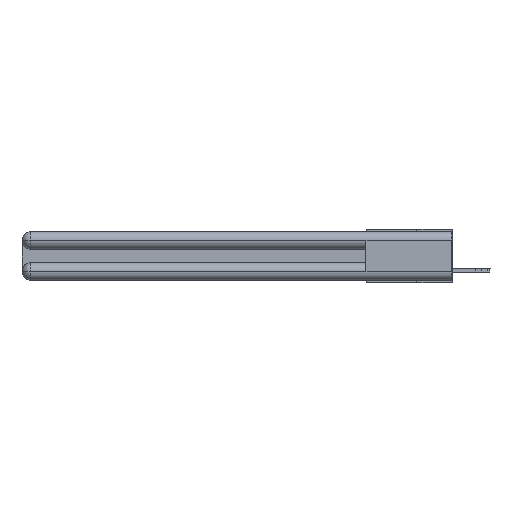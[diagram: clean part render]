
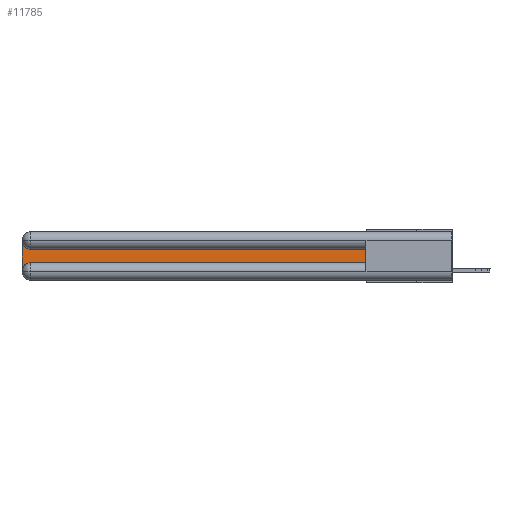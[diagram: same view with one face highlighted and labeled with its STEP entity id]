
A CAD part, left-side view. The second image highlights one B-rep face of the part: STEP entity #11785.
In plain terms, the highlighted planar face has unit normal (-1, 0, 0).
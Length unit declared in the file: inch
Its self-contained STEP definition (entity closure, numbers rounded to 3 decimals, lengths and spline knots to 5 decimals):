
#1414 = VERTEX_POINT ( 'NONE', #13036 ) ;
#1997 = LINE ( 'NONE', #21992, #21775 ) ;
#3199 = EDGE_CURVE ( 'NONE', #17450, #18612, #3644, .T. ) ;
#3342 = AXIS2_PLACEMENT_3D ( 'NONE', #25469, #17498, #21506 ) ;
#3433 = EDGE_LOOP ( 'NONE', ( #16272, #20812, #24108, #17010, #16637, #19248 ) ) ;
#3644 = LINE ( 'NONE', #16862, #15412 ) ;
#3791 = DIRECTION ( 'NONE',  ( 0., 0., -1. ) ) ;
#3910 = DIRECTION ( 'NONE',  ( 1., 0., 0. ) ) ;
#4842 = AXIS2_PLACEMENT_3D ( 'NONE', #20042, #3910, #5794 ) ;
#4911 = EDGE_CURVE ( 'NONE', #5305, #17450, #18140, .T. ) ;
#5305 = VERTEX_POINT ( 'NONE', #14785 ) ;
#5508 = CARTESIAN_POINT ( 'NONE',  ( 0.075, 2.94, -0.2775 ) ) ;
#5794 = DIRECTION ( 'NONE',  ( 0., 0., -1. ) ) ;
#6445 = CIRCLE ( 'NONE', #13655, 0.06 ) ;
#6840 = CARTESIAN_POINT ( 'NONE',  ( 0.075, 0.6, -0.2175 ) ) ;
#7050 = VERTEX_POINT ( 'NONE', #12999 ) ;
#8280 = VECTOR ( 'NONE', #10833, 39.37008 ) ;
#8893 = VECTOR ( 'NONE', #21657, 39.37008 ) ;
#9766 = PLANE ( 'NONE',  #4842 ) ;
#9778 = CARTESIAN_POINT ( 'NONE',  ( 0.075, 2.94, -0.2175 ) ) ;
#10819 = DIRECTION ( 'NONE',  ( 0., 1., 0. ) ) ;
#10833 = DIRECTION ( 'NONE',  ( 0., 0., 1. ) ) ;
#11087 = VERTEX_POINT ( 'NONE', #9778 ) ;
#11785 = ADVANCED_FACE ( 'NONE', ( #13609 ), #9766, .F. ) ;
#12999 = CARTESIAN_POINT ( 'NONE',  ( 0.075, 3., -0.0625 ) ) ;
#13036 = CARTESIAN_POINT ( 'NONE',  ( 0.075, 3., -0.2775 ) ) ;
#13304 = CARTESIAN_POINT ( 'NONE',  ( 0.075, 2.94, -0.1225 ) ) ;
#13609 = FACE_OUTER_BOUND ( 'NONE', #3433, .T. ) ;
#13655 = AXIS2_PLACEMENT_3D ( 'NONE', #5508, #25874, #15913 ) ;
#13924 = LINE ( 'NONE', #15565, #8893 ) ;
#14785 = CARTESIAN_POINT ( 'NONE',  ( 0.075, 0.6, -0.2175 ) ) ;
#15412 = VECTOR ( 'NONE', #10819, 39.37008 ) ;
#15565 = CARTESIAN_POINT ( 'NONE',  ( 0.075, 0.6, -0.2175 ) ) ;
#15913 = DIRECTION ( 'NONE',  ( 0., 0., -1. ) ) ;
#16272 = ORIENTED_EDGE ( 'NONE', *, *, #3199, .T. ) ;
#16637 = ORIENTED_EDGE ( 'NONE', *, *, #22277, .T. ) ;
#16862 = CARTESIAN_POINT ( 'NONE',  ( 0.075, 0.6, -0.1225 ) ) ;
#17010 = ORIENTED_EDGE ( 'NONE', *, *, #24891, .T. ) ;
#17450 = VERTEX_POINT ( 'NONE', #21426 ) ;
#17498 = DIRECTION ( 'NONE',  ( 1., 0., 0. ) ) ;
#18140 = LINE ( 'NONE', #6840, #8280 ) ;
#18612 = VERTEX_POINT ( 'NONE', #13304 ) ;
#19248 = ORIENTED_EDGE ( 'NONE', *, *, #4911, .T. ) ;
#19491 = EDGE_CURVE ( 'NONE', #7050, #1414, #1997, .T. ) ;
#20042 = CARTESIAN_POINT ( 'NONE',  ( 0.075, 3., -0.1225 ) ) ;
#20812 = ORIENTED_EDGE ( 'NONE', *, *, #21091, .T. ) ;
#21055 = CIRCLE ( 'NONE', #3342, 0.06 ) ;
#21091 = EDGE_CURVE ( 'NONE', #18612, #7050, #21055, .T. ) ;
#21426 = CARTESIAN_POINT ( 'NONE',  ( 0.075, 0.6, -0.1225 ) ) ;
#21506 = DIRECTION ( 'NONE',  ( 0., 0., -1. ) ) ;
#21657 = DIRECTION ( 'NONE',  ( 0., -1., 0. ) ) ;
#21775 = VECTOR ( 'NONE', #3791, 39.37008 ) ;
#21992 = CARTESIAN_POINT ( 'NONE',  ( 0.075, 3., -0.2175 ) ) ;
#22277 = EDGE_CURVE ( 'NONE', #11087, #5305, #13924, .T. ) ;
#24108 = ORIENTED_EDGE ( 'NONE', *, *, #19491, .T. ) ;
#24891 = EDGE_CURVE ( 'NONE', #1414, #11087, #6445, .T. ) ;
#25469 = CARTESIAN_POINT ( 'NONE',  ( 0.075, 2.94, -0.0625 ) ) ;
#25874 = DIRECTION ( 'NONE',  ( 1., 0., 0. ) ) ;
